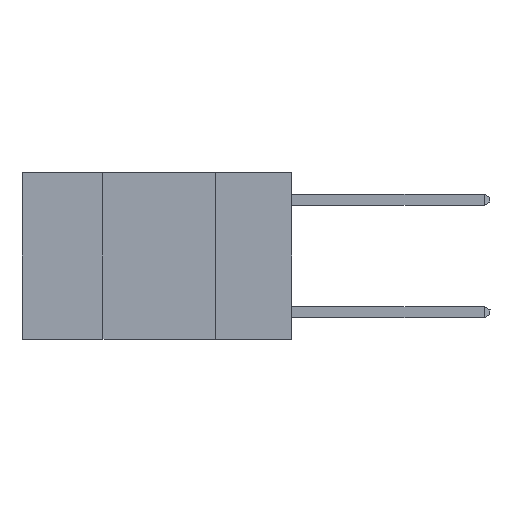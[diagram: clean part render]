
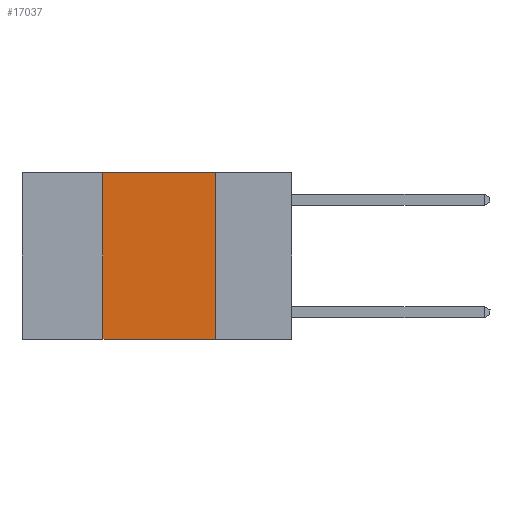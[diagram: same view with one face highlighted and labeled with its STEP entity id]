
A CAD part, left-side view. The second image highlights one B-rep face of the part: STEP entity #17037.
In plain terms, the highlighted planar face has unit normal (-1, 0, 0).
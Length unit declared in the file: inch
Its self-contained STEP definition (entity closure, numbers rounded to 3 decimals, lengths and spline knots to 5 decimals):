
#574 = VERTEX_POINT ( 'NONE', #12391 ) ;
#1069 = VECTOR ( 'NONE', #14264, 39.37008 ) ;
#1250 = LINE ( 'NONE', #17834, #13965 ) ;
#1381 = PLANE ( 'NONE',  #13278 ) ;
#1604 = LINE ( 'NONE', #7858, #1069 ) ;
#2362 = EDGE_CURVE ( 'NONE', #574, #8205, #1604, .T. ) ;
#2925 = VECTOR ( 'NONE', #13955, 39.37008 ) ;
#2974 = EDGE_CURVE ( 'NONE', #9113, #3857, #12323, .T. ) ;
#3112 = DIRECTION ( 'NONE',  ( 0., 0., -1. ) ) ;
#3857 = VERTEX_POINT ( 'NONE', #9744 ) ;
#4747 = CARTESIAN_POINT ( 'NONE',  ( 0., 0.6, 0. ) ) ;
#5404 = CARTESIAN_POINT ( 'NONE',  ( 0., 0.42, -0.37 ) ) ;
#5998 = ORIENTED_EDGE ( 'NONE', *, *, #18264, .T. ) ;
#7765 = ORIENTED_EDGE ( 'NONE', *, *, #2362, .F. ) ;
#7858 = CARTESIAN_POINT ( 'NONE',  ( 0., 0.17, 0. ) ) ;
#8201 = EDGE_LOOP ( 'NONE', ( #7765, #18617, #12640, #5998 ) ) ;
#8205 = VERTEX_POINT ( 'NONE', #9140 ) ;
#8279 = FACE_OUTER_BOUND ( 'NONE', #8201, .T. ) ;
#9113 = VERTEX_POINT ( 'NONE', #5404 ) ;
#9140 = CARTESIAN_POINT ( 'NONE',  ( 0., 0.17, -0.37 ) ) ;
#9744 = CARTESIAN_POINT ( 'NONE',  ( 0., 0.42, 0. ) ) ;
#11233 = VECTOR ( 'NONE', #16155, 39.37008 ) ;
#11763 = LINE ( 'NONE', #17633, #11233 ) ;
#12323 = LINE ( 'NONE', #18671, #2925 ) ;
#12391 = CARTESIAN_POINT ( 'NONE',  ( 0., 0.17, 0. ) ) ;
#12640 = ORIENTED_EDGE ( 'NONE', *, *, #2974, .F. ) ;
#13067 = DIRECTION ( 'NONE',  ( 1., 0., 0. ) ) ;
#13278 = AXIS2_PLACEMENT_3D ( 'NONE', #4747, #13067, #3112 ) ;
#13955 = DIRECTION ( 'NONE',  ( 0., 0., 1. ) ) ;
#13965 = VECTOR ( 'NONE', #19389, 39.37008 ) ;
#14264 = DIRECTION ( 'NONE',  ( 0., 0., -1. ) ) ;
#16155 = DIRECTION ( 'NONE',  ( 0., -1., 0. ) ) ;
#17037 = ADVANCED_FACE ( 'NONE', ( #8279 ), #1381, .F. ) ;
#17633 = CARTESIAN_POINT ( 'NONE',  ( 0., 0.6, -0.37 ) ) ;
#17834 = CARTESIAN_POINT ( 'NONE',  ( 0., 0.6, 0. ) ) ;
#18264 = EDGE_CURVE ( 'NONE', #9113, #8205, #11763, .T. ) ;
#18343 = EDGE_CURVE ( 'NONE', #3857, #574, #1250, .T. ) ;
#18617 = ORIENTED_EDGE ( 'NONE', *, *, #18343, .F. ) ;
#18671 = CARTESIAN_POINT ( 'NONE',  ( 0., 0.42, 0. ) ) ;
#19389 = DIRECTION ( 'NONE',  ( 0., -1., 0. ) ) ;
